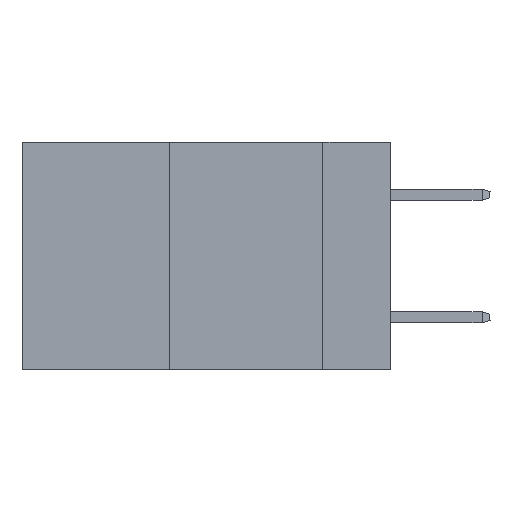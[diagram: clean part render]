
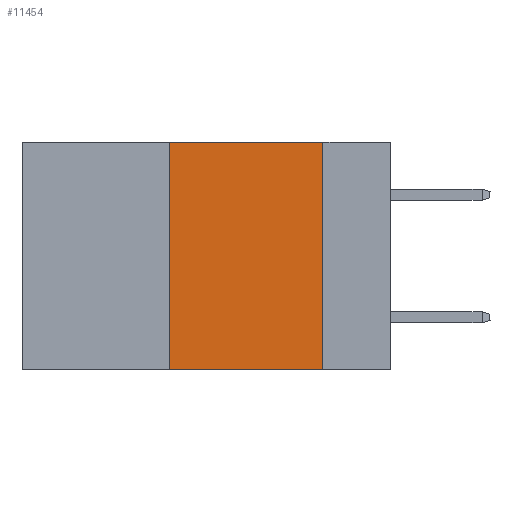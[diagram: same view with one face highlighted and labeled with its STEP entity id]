
A CAD part, left-side view. The second image highlights one B-rep face of the part: STEP entity #11454.
In plain terms, the highlighted planar face has unit normal (-1, 0, 0).
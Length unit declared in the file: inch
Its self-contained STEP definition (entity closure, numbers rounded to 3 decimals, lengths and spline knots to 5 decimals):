
#751 = CARTESIAN_POINT ( 'NONE',  ( 0., 0.36, -0.37 ) ) ;
#1423 = CARTESIAN_POINT ( 'NONE',  ( 0., 0.36, 0. ) ) ;
#1769 = CARTESIAN_POINT ( 'NONE',  ( 0., 0.6, -0.37 ) ) ;
#3242 = CARTESIAN_POINT ( 'NONE',  ( 0., 0.6, 0. ) ) ;
#3249 = CARTESIAN_POINT ( 'NONE',  ( 0., 0.6, 0. ) ) ;
#3720 = DIRECTION ( 'NONE',  ( 0., -1., 0. ) ) ;
#5109 = AXIS2_PLACEMENT_3D ( 'NONE', #3249, #16586, #5198 ) ;
#5198 = DIRECTION ( 'NONE',  ( 0., 0., -1. ) ) ;
#5838 = DIRECTION ( 'NONE',  ( 0., 0., 1. ) ) ;
#5896 = VERTEX_POINT ( 'NONE', #22722 ) ;
#6776 = ORIENTED_EDGE ( 'NONE', *, *, #14131, .F. ) ;
#6960 = VECTOR ( 'NONE', #3720, 39.37008 ) ;
#7747 = VECTOR ( 'NONE', #22278, 39.37008 ) ;
#8320 = LINE ( 'NONE', #20387, #7747 ) ;
#8569 = LINE ( 'NONE', #3242, #22502 ) ;
#9474 = LINE ( 'NONE', #19108, #23353 ) ;
#10337 = ORIENTED_EDGE ( 'NONE', *, *, #19753, .F. ) ;
#11454 = ADVANCED_FACE ( 'NONE', ( #18831 ), #22153, .F. ) ;
#11938 = CARTESIAN_POINT ( 'NONE',  ( 0., 0.11, 0. ) ) ;
#12219 = EDGE_CURVE ( 'NONE', #21862, #5896, #22057, .T. ) ;
#12440 = VERTEX_POINT ( 'NONE', #11938 ) ;
#14131 = EDGE_CURVE ( 'NONE', #12440, #5896, #8320, .T. ) ;
#14152 = VERTEX_POINT ( 'NONE', #1423 ) ;
#15715 = ORIENTED_EDGE ( 'NONE', *, *, #12219, .T. ) ;
#16586 = DIRECTION ( 'NONE',  ( 1., 0., 0. ) ) ;
#16738 = EDGE_LOOP ( 'NONE', ( #6776, #10337, #20410, #15715 ) ) ;
#18462 = DIRECTION ( 'NONE',  ( 0., -1., 0. ) ) ;
#18831 = FACE_OUTER_BOUND ( 'NONE', #16738, .T. ) ;
#19108 = CARTESIAN_POINT ( 'NONE',  ( 0., 0.36, 0. ) ) ;
#19753 = EDGE_CURVE ( 'NONE', #14152, #12440, #8569, .T. ) ;
#19971 = EDGE_CURVE ( 'NONE', #21862, #14152, #9474, .T. ) ;
#20387 = CARTESIAN_POINT ( 'NONE',  ( 0., 0.11, 0. ) ) ;
#20410 = ORIENTED_EDGE ( 'NONE', *, *, #19971, .F. ) ;
#21862 = VERTEX_POINT ( 'NONE', #751 ) ;
#22057 = LINE ( 'NONE', #1769, #6960 ) ;
#22153 = PLANE ( 'NONE',  #5109 ) ;
#22278 = DIRECTION ( 'NONE',  ( 0., 0., -1. ) ) ;
#22502 = VECTOR ( 'NONE', #18462, 39.37008 ) ;
#22722 = CARTESIAN_POINT ( 'NONE',  ( 0., 0.11, -0.37 ) ) ;
#23353 = VECTOR ( 'NONE', #5838, 39.37008 ) ;
